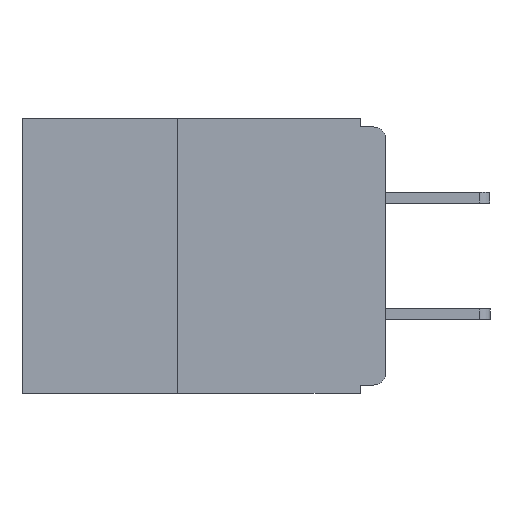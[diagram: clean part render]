
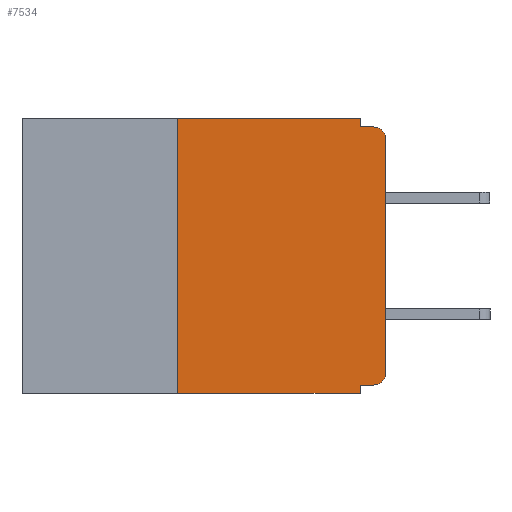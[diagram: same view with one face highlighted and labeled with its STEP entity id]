
A CAD part, left-side view. The second image highlights one B-rep face of the part: STEP entity #7534.
In plain terms, the highlighted planar face has unit normal (-1, 0, 0).
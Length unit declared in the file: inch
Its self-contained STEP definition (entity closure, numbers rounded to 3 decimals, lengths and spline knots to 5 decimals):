
#7 = LINE ( 'NONE', #9929, #12845 ) ;
#194 = ORIENTED_EDGE ( 'NONE', *, *, #7476, .F. ) ;
#271 = CARTESIAN_POINT ( 'NONE',  ( 0., 0., -0.305 ) ) ;
#335 = LINE ( 'NONE', #5332, #15678 ) ;
#451 = ORIENTED_EDGE ( 'NONE', *, *, #4504, .F. ) ;
#639 = CARTESIAN_POINT ( 'NONE',  ( 0., 0.25, 0. ) ) ;
#648 = CARTESIAN_POINT ( 'NONE',  ( 0., 0.437, 0. ) ) ;
#675 = DIRECTION ( 'NONE',  ( 0., -1., 0. ) ) ;
#781 = FACE_OUTER_BOUND ( 'NONE', #9894, .T. ) ;
#985 = CARTESIAN_POINT ( 'NONE',  ( 0., 0.437, -0.33 ) ) ;
#1597 = DIRECTION ( 'NONE',  ( 0., 0., 1. ) ) ;
#1893 = EDGE_CURVE ( 'NONE', #2470, #2455, #335, .T. ) ;
#2112 = DIRECTION ( 'NONE',  ( 0., 0., -1. ) ) ;
#2455 = VERTEX_POINT ( 'NONE', #11722 ) ;
#2470 = VERTEX_POINT ( 'NONE', #271 ) ;
#2648 = AXIS2_PLACEMENT_3D ( 'NONE', #14627, #15518, #15290 ) ;
#2892 = ORIENTED_EDGE ( 'NONE', *, *, #5266, .T. ) ;
#3096 = LINE ( 'NONE', #9323, #14755 ) ;
#3335 = CIRCLE ( 'NONE', #10469, 0.015 ) ;
#3417 = ORIENTED_EDGE ( 'NONE', *, *, #11211, .F. ) ;
#3536 = EDGE_CURVE ( 'NONE', #13768, #13455, #14085, .T. ) ;
#4020 = DIRECTION ( 'NONE',  ( 0., 0., -1. ) ) ;
#4037 = DIRECTION ( 'NONE',  ( -1., 0., 0. ) ) ;
#4053 = CARTESIAN_POINT ( 'NONE',  ( 0., 0.015, -0.025 ) ) ;
#4504 = EDGE_CURVE ( 'NONE', #14865, #13768, #3096, .T. ) ;
#4946 = EDGE_CURVE ( 'NONE', #5535, #10284, #6145, .T. ) ;
#5056 = VECTOR ( 'NONE', #675, 39.37008 ) ;
#5228 = CARTESIAN_POINT ( 'NONE',  ( 0., 0.25, -0.33 ) ) ;
#5266 = EDGE_CURVE ( 'NONE', #14865, #2470, #8060, .T. ) ;
#5332 = CARTESIAN_POINT ( 'NONE',  ( 0., 0., 0. ) ) ;
#5364 = ORIENTED_EDGE ( 'NONE', *, *, #11050, .F. ) ;
#5535 = VERTEX_POINT ( 'NONE', #5228 ) ;
#5540 = DIRECTION ( 'NONE',  ( -1., 0., 0. ) ) ;
#5936 = VERTEX_POINT ( 'NONE', #14867 ) ;
#6145 = LINE ( 'NONE', #14788, #8996 ) ;
#6286 = ORIENTED_EDGE ( 'NONE', *, *, #1893, .T. ) ;
#6331 = ORIENTED_EDGE ( 'NONE', *, *, #3536, .F. ) ;
#6921 = VERTEX_POINT ( 'NONE', #11430 ) ;
#6956 = DIRECTION ( 'NONE',  ( 0., 0., -1. ) ) ;
#7303 = CARTESIAN_POINT ( 'NONE',  ( 0., 0.031, -0.33 ) ) ;
#7476 = EDGE_CURVE ( 'NONE', #10284, #6921, #14494, .T. ) ;
#7534 = ADVANCED_FACE ( 'NONE', ( #781 ), #13796, .F. ) ;
#7865 = ORIENTED_EDGE ( 'NONE', *, *, #12957, .T. ) ;
#8060 = CIRCLE ( 'NONE', #12091, 0.015 ) ;
#8111 = DIRECTION ( 'NONE',  ( 0., 1., 0. ) ) ;
#8490 = VERTEX_POINT ( 'NONE', #14161 ) ;
#8708 = CARTESIAN_POINT ( 'NONE',  ( 0., 0.015, -0.32 ) ) ;
#8996 = VECTOR ( 'NONE', #1597, 39.37008 ) ;
#9133 = ORIENTED_EDGE ( 'NONE', *, *, #9839, .T. ) ;
#9196 = CARTESIAN_POINT ( 'NONE',  ( 0., 0.015, -0.305 ) ) ;
#9261 = LINE ( 'NONE', #985, #12055 ) ;
#9323 = CARTESIAN_POINT ( 'NONE',  ( 0., 0., -0.32 ) ) ;
#9499 = ORIENTED_EDGE ( 'NONE', *, *, #4946, .F. ) ;
#9839 = EDGE_CURVE ( 'NONE', #2455, #8490, #3335, .T. ) ;
#9872 = CARTESIAN_POINT ( 'NONE',  ( 0., 0.031, -0.32 ) ) ;
#9894 = EDGE_LOOP ( 'NONE', ( #6286, #9133, #3417, #5364, #194, #9499, #7865, #6331, #451, #2892 ) ) ;
#9929 = CARTESIAN_POINT ( 'NONE',  ( 0., 0., -0.01 ) ) ;
#10051 = DIRECTION ( 'NONE',  ( 0., 0., 1. ) ) ;
#10284 = VERTEX_POINT ( 'NONE', #639 ) ;
#10469 = AXIS2_PLACEMENT_3D ( 'NONE', #4053, #4037, #4020 ) ;
#10823 = CARTESIAN_POINT ( 'NONE',  ( 0., 0.031, 0. ) ) ;
#11050 = EDGE_CURVE ( 'NONE', #6921, #5936, #14874, .T. ) ;
#11211 = EDGE_CURVE ( 'NONE', #5936, #8490, #7, .T. ) ;
#11430 = CARTESIAN_POINT ( 'NONE',  ( 0., 0.031, 0. ) ) ;
#11722 = CARTESIAN_POINT ( 'NONE',  ( 0., 0., -0.025 ) ) ;
#11896 = DIRECTION ( 'NONE',  ( 0., 0., -1. ) ) ;
#11926 = VECTOR ( 'NONE', #2112, 39.37008 ) ;
#12055 = VECTOR ( 'NONE', #13272, 39.37008 ) ;
#12091 = AXIS2_PLACEMENT_3D ( 'NONE', #9196, #5540, #6956 ) ;
#12845 = VECTOR ( 'NONE', #13401, 39.37008 ) ;
#12957 = EDGE_CURVE ( 'NONE', #5535, #13455, #9261, .T. ) ;
#13168 = CARTESIAN_POINT ( 'NONE',  ( 0., 0.031, -0.33 ) ) ;
#13272 = DIRECTION ( 'NONE',  ( 0., -1., 0. ) ) ;
#13401 = DIRECTION ( 'NONE',  ( 0., -1., 0. ) ) ;
#13424 = VECTOR ( 'NONE', #11896, 39.37008 ) ;
#13455 = VERTEX_POINT ( 'NONE', #13168 ) ;
#13768 = VERTEX_POINT ( 'NONE', #9872 ) ;
#13796 = PLANE ( 'NONE',  #2648 ) ;
#14085 = LINE ( 'NONE', #7303, #13424 ) ;
#14161 = CARTESIAN_POINT ( 'NONE',  ( 0., 0.015, -0.01 ) ) ;
#14494 = LINE ( 'NONE', #648, #5056 ) ;
#14627 = CARTESIAN_POINT ( 'NONE',  ( 0., 0.437, 0. ) ) ;
#14755 = VECTOR ( 'NONE', #8111, 39.37008 ) ;
#14788 = CARTESIAN_POINT ( 'NONE',  ( 0., 0.25, -0.33 ) ) ;
#14865 = VERTEX_POINT ( 'NONE', #8708 ) ;
#14867 = CARTESIAN_POINT ( 'NONE',  ( 0., 0.031, -0.01 ) ) ;
#14874 = LINE ( 'NONE', #10823, #11926 ) ;
#15290 = DIRECTION ( 'NONE',  ( 0., 0., -1. ) ) ;
#15518 = DIRECTION ( 'NONE',  ( 1., 0., 0. ) ) ;
#15678 = VECTOR ( 'NONE', #10051, 39.37008 ) ;
